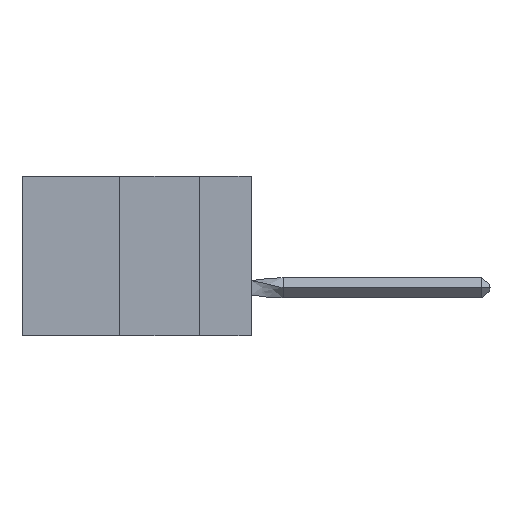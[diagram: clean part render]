
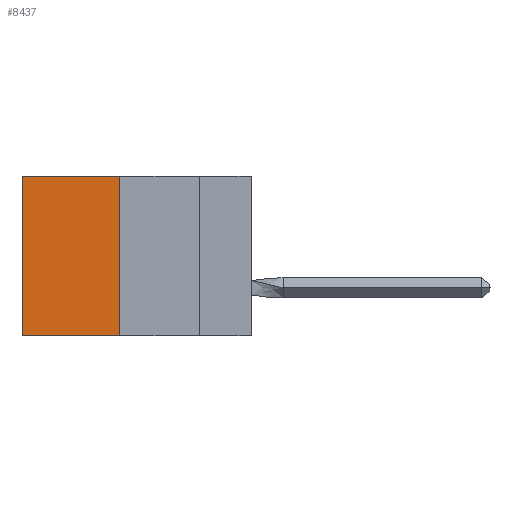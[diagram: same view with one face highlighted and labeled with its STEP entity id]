
A CAD part, left-side view. The second image highlights one B-rep face of the part: STEP entity #8437.
In plain terms, the highlighted planar face has unit normal (-1, 0, 0).
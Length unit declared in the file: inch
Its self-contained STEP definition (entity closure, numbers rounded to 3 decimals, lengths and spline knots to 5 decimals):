
#1443 = EDGE_CURVE ( 'NONE', #3666, #5808, #13924, .T. ) ;
#1814 = EDGE_CURVE ( 'NONE', #5808, #22956, #13599, .T. ) ;
#1892 = CARTESIAN_POINT ( 'NONE',  ( 0.305, 0.413, 0. ) ) ;
#3666 = VERTEX_POINT ( 'NONE', #1892 ) ;
#5521 = PLANE ( 'NONE',  #14384 ) ;
#5808 = VERTEX_POINT ( 'NONE', #6086 ) ;
#5909 = DIRECTION ( 'NONE',  ( 0., 0., -1. ) ) ;
#5990 = EDGE_LOOP ( 'NONE', ( #9708, #6761, #13531, #7615 ) ) ;
#6086 = CARTESIAN_POINT ( 'NONE',  ( 0.305, 0.72, 0. ) ) ;
#6089 = VECTOR ( 'NONE', #5909, 39.37008 ) ;
#6383 = FACE_OUTER_BOUND ( 'NONE', #5990, .T. ) ;
#6442 = LINE ( 'NONE', #19229, #13400 ) ;
#6761 = ORIENTED_EDGE ( 'NONE', *, *, #17190, .F. ) ;
#7615 = ORIENTED_EDGE ( 'NONE', *, *, #1443, .T. ) ;
#7890 = LINE ( 'NONE', #23336, #6089 ) ;
#8437 = ADVANCED_FACE ( 'NONE', ( #6383 ), #5521, .F. ) ;
#8459 = VECTOR ( 'NONE', #16443, 39.37008 ) ;
#8615 = CARTESIAN_POINT ( 'NONE',  ( 0.305, 0.72, -0.5 ) ) ;
#9708 = ORIENTED_EDGE ( 'NONE', *, *, #1814, .T. ) ;
#11357 = CARTESIAN_POINT ( 'NONE',  ( 0.305, 0.413, 0. ) ) ;
#12205 = CARTESIAN_POINT ( 'NONE',  ( 0.305, 0.72, -0.5 ) ) ;
#12949 = DIRECTION ( 'NONE',  ( 0., 1., 0. ) ) ;
#13400 = VECTOR ( 'NONE', #20665, 39.37008 ) ;
#13531 = ORIENTED_EDGE ( 'NONE', *, *, #18843, .F. ) ;
#13599 = LINE ( 'NONE', #8615, #8459 ) ;
#13924 = LINE ( 'NONE', #11357, #15785 ) ;
#14384 = AXIS2_PLACEMENT_3D ( 'NONE', #19086, #17238, #21061 ) ;
#14545 = CARTESIAN_POINT ( 'NONE',  ( 0.305, 0.413, -0.5 ) ) ;
#15785 = VECTOR ( 'NONE', #12949, 39.37008 ) ;
#16443 = DIRECTION ( 'NONE',  ( 0., 0., -1. ) ) ;
#17190 = EDGE_CURVE ( 'NONE', #19834, #22956, #6442, .T. ) ;
#17238 = DIRECTION ( 'NONE',  ( 1., 0., 0. ) ) ;
#18843 = EDGE_CURVE ( 'NONE', #3666, #19834, #7890, .T. ) ;
#19086 = CARTESIAN_POINT ( 'NONE',  ( 0.305, 0.413, -0.5 ) ) ;
#19229 = CARTESIAN_POINT ( 'NONE',  ( 0.305, 0.413, -0.5 ) ) ;
#19834 = VERTEX_POINT ( 'NONE', #14545 ) ;
#20665 = DIRECTION ( 'NONE',  ( 0., 1., 0. ) ) ;
#21061 = DIRECTION ( 'NONE',  ( 0., 0., -1. ) ) ;
#22956 = VERTEX_POINT ( 'NONE', #12205 ) ;
#23336 = CARTESIAN_POINT ( 'NONE',  ( 0.305, 0.413, -0.5 ) ) ;
